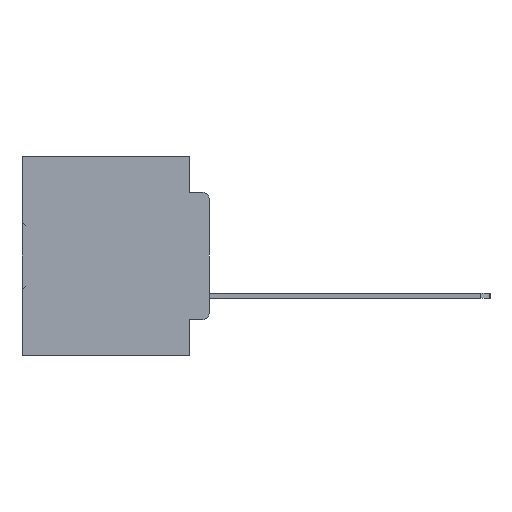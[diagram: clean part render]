
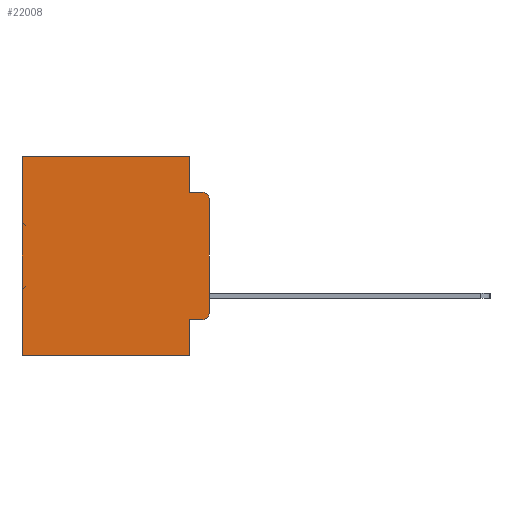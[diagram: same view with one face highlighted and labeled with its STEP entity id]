
A CAD part, left-side view. The second image highlights one B-rep face of the part: STEP entity #22008.
In plain terms, the highlighted planar face has unit normal (-1, 0, 0).
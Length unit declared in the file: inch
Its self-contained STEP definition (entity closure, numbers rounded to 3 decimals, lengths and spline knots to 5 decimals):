
#168 = ORIENTED_EDGE ( 'NONE', *, *, #23469, .F. ) ;
#632 = VECTOR ( 'NONE', #8751, 39.37008 ) ;
#692 = FACE_OUTER_BOUND ( 'NONE', #12632, .T. ) ;
#705 = ORIENTED_EDGE ( 'NONE', *, *, #16900, .F. ) ;
#1130 = CARTESIAN_POINT ( 'NONE',  ( 0.298, 0., -0.5 ) ) ;
#3029 = CARTESIAN_POINT ( 'NONE',  ( 0.298, 0.051, -0.5 ) ) ;
#3193 = VERTEX_POINT ( 'NONE', #22056 ) ;
#3244 = CARTESIAN_POINT ( 'NONE',  ( 0.298, 0.051, -0.0885 ) ) ;
#3470 = CARTESIAN_POINT ( 'NONE',  ( 0.298, 0.02, -0.4115 ) ) ;
#3932 = CARTESIAN_POINT ( 'NONE',  ( 0.298, 0.051, -0.4115 ) ) ;
#4107 = EDGE_CURVE ( 'NONE', #3193, #8709, #20814, .T. ) ;
#4770 = DIRECTION ( 'NONE',  ( 0., 0., -1. ) ) ;
#5457 = ORIENTED_EDGE ( 'NONE', *, *, #29557, .T. ) ;
#6289 = DIRECTION ( 'NONE',  ( -1., 0., 0. ) ) ;
#6812 = DIRECTION ( 'NONE',  ( 0., 1., 0. ) ) ;
#7404 = VECTOR ( 'NONE', #15262, 39.37008 ) ;
#7479 = CARTESIAN_POINT ( 'NONE',  ( 0.298, 0.02, -0.3915 ) ) ;
#7808 = CARTESIAN_POINT ( 'NONE',  ( 0.298, 0.051, 0. ) ) ;
#7837 = ORIENTED_EDGE ( 'NONE', *, *, #28116, .F. ) ;
#7948 = CARTESIAN_POINT ( 'NONE',  ( 0.298, 0.051, 0. ) ) ;
#8333 = LINE ( 'NONE', #23104, #632 ) ;
#8348 = ORIENTED_EDGE ( 'NONE', *, *, #25235, .F. ) ;
#8533 = EDGE_CURVE ( 'NONE', #3193, #17529, #9268, .T. ) ;
#8709 = VERTEX_POINT ( 'NONE', #33123 ) ;
#8751 = DIRECTION ( 'NONE',  ( 0., -1., 0. ) ) ;
#9115 = VECTOR ( 'NONE', #6812, 39.37008 ) ;
#9155 = LINE ( 'NONE', #11608, #15987 ) ;
#9268 = LINE ( 'NONE', #9412, #7404 ) ;
#9412 = CARTESIAN_POINT ( 'NONE',  ( 0.298, 0., 0. ) ) ;
#9946 = EDGE_CURVE ( 'NONE', #12061, #17529, #29468, .T. ) ;
#10038 = LINE ( 'NONE', #1130, #9115 ) ;
#10468 = DIRECTION ( 'NONE',  ( 0., 0., -1. ) ) ;
#10805 = DIRECTION ( 'NONE',  ( 0., 0., -1. ) ) ;
#10836 = CARTESIAN_POINT ( 'NONE',  ( 0.298, 0.473, -0.5 ) ) ;
#11608 = CARTESIAN_POINT ( 'NONE',  ( 0.298, 0., 0. ) ) ;
#11718 = AXIS2_PLACEMENT_3D ( 'NONE', #23602, #6289, #26437 ) ;
#12029 = LINE ( 'NONE', #7808, #26311 ) ;
#12061 = VERTEX_POINT ( 'NONE', #3470 ) ;
#12632 = EDGE_LOOP ( 'NONE', ( #16447, #21121, #168, #705, #15571, #19280, #8348, #7837, #5457, #34480 ) ) ;
#12845 = VECTOR ( 'NONE', #18403, 39.37008 ) ;
#13468 = DIRECTION ( 'NONE',  ( 0., 0., -1. ) ) ;
#13760 = VERTEX_POINT ( 'NONE', #10836 ) ;
#15262 = DIRECTION ( 'NONE',  ( 0., 0., -1. ) ) ;
#15571 = ORIENTED_EDGE ( 'NONE', *, *, #18201, .T. ) ;
#15806 = VERTEX_POINT ( 'NONE', #3029 ) ;
#15987 = VECTOR ( 'NONE', #28662, 39.37008 ) ;
#16447 = ORIENTED_EDGE ( 'NONE', *, *, #8533, .F. ) ;
#16900 = EDGE_CURVE ( 'NONE', #28613, #24167, #12029, .T. ) ;
#17529 = VERTEX_POINT ( 'NONE', #25033 ) ;
#18201 = EDGE_CURVE ( 'NONE', #28613, #22836, #9155, .T. ) ;
#18403 = DIRECTION ( 'NONE',  ( 0., -1., 0. ) ) ;
#18635 = EDGE_CURVE ( 'NONE', #22836, #13760, #31488, .T. ) ;
#19280 = ORIENTED_EDGE ( 'NONE', *, *, #18635, .T. ) ;
#20814 = CIRCLE ( 'NONE', #11718, 0.02 ) ;
#21121 = ORIENTED_EDGE ( 'NONE', *, *, #4107, .T. ) ;
#21279 = VERTEX_POINT ( 'NONE', #28661 ) ;
#21537 = LINE ( 'NONE', #36909, #34680 ) ;
#21960 = PLANE ( 'NONE',  #26470 ) ;
#22008 = ADVANCED_FACE ( 'NONE', ( #692 ), #21960, .F. ) ;
#22056 = CARTESIAN_POINT ( 'NONE',  ( 0.298, 0., -0.1085 ) ) ;
#22836 = VERTEX_POINT ( 'NONE', #33799 ) ;
#23104 = CARTESIAN_POINT ( 'NONE',  ( 0.298, 0.051, -0.0885 ) ) ;
#23469 = EDGE_CURVE ( 'NONE', #24167, #8709, #8333, .T. ) ;
#23602 = CARTESIAN_POINT ( 'NONE',  ( 0.298, 0.02, -0.1085 ) ) ;
#24013 = VECTOR ( 'NONE', #4770, 39.37008 ) ;
#24167 = VERTEX_POINT ( 'NONE', #3244 ) ;
#25033 = CARTESIAN_POINT ( 'NONE',  ( 0.298, 0., -0.3915 ) ) ;
#25235 = EDGE_CURVE ( 'NONE', #15806, #13760, #10038, .T. ) ;
#26311 = VECTOR ( 'NONE', #10805, 39.37008 ) ;
#26437 = DIRECTION ( 'NONE',  ( 0., 0., -1. ) ) ;
#26470 = AXIS2_PLACEMENT_3D ( 'NONE', #35911, #30452, #13468 ) ;
#27570 = DIRECTION ( 'NONE',  ( -1., 0., 0. ) ) ;
#27657 = CARTESIAN_POINT ( 'NONE',  ( 0.298, 0.473, 0. ) ) ;
#28116 = EDGE_CURVE ( 'NONE', #21279, #15806, #21537, .T. ) ;
#28613 = VERTEX_POINT ( 'NONE', #7948 ) ;
#28661 = CARTESIAN_POINT ( 'NONE',  ( 0.298, 0.051, -0.4115 ) ) ;
#28662 = DIRECTION ( 'NONE',  ( 0., 1., 0. ) ) ;
#28862 = LINE ( 'NONE', #3932, #12845 ) ;
#29468 = CIRCLE ( 'NONE', #30659, 0.02 ) ;
#29557 = EDGE_CURVE ( 'NONE', #21279, #12061, #28862, .T. ) ;
#30452 = DIRECTION ( 'NONE',  ( 1., 0., 0. ) ) ;
#30659 = AXIS2_PLACEMENT_3D ( 'NONE', #7479, #27570, #10468 ) ;
#31488 = LINE ( 'NONE', #27657, #24013 ) ;
#33123 = CARTESIAN_POINT ( 'NONE',  ( 0.298, 0.02, -0.0885 ) ) ;
#33799 = CARTESIAN_POINT ( 'NONE',  ( 0.298, 0.473, 0. ) ) ;
#34480 = ORIENTED_EDGE ( 'NONE', *, *, #9946, .T. ) ;
#34680 = VECTOR ( 'NONE', #36805, 39.37008 ) ;
#35911 = CARTESIAN_POINT ( 'NONE',  ( 0.298, 0., 0. ) ) ;
#36805 = DIRECTION ( 'NONE',  ( 0., 0., -1. ) ) ;
#36909 = CARTESIAN_POINT ( 'NONE',  ( 0.298, 0.051, 0. ) ) ;
